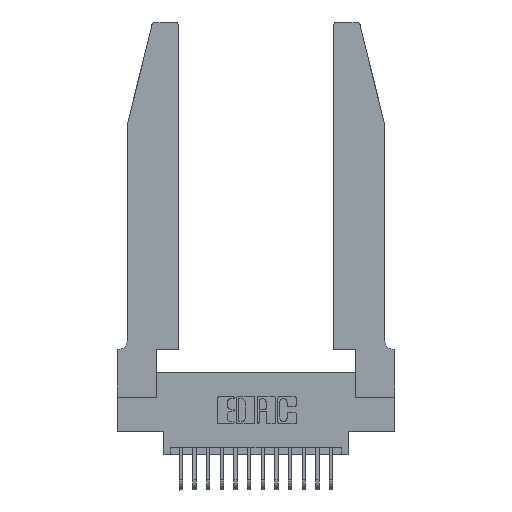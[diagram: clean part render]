
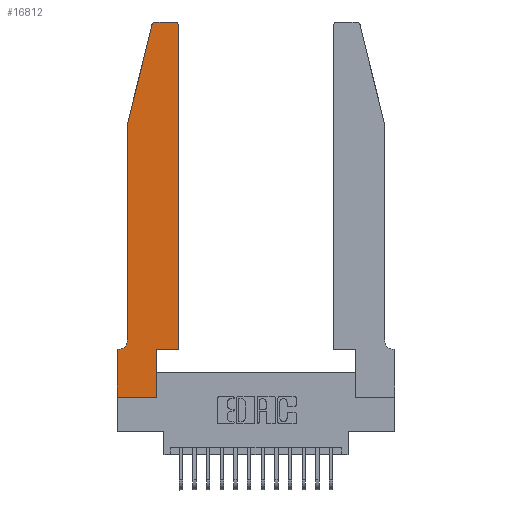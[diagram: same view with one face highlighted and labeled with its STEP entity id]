
A CAD part, top view. The second image highlights one B-rep face of the part: STEP entity #16812.
In plain terms, the highlighted planar face has unit normal (0, 0, 1).
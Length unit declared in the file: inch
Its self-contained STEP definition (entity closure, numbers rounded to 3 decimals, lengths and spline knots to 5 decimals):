
#8 = AXIS2_PLACEMENT_3D ( 'NONE', #12421, #4055, #13852 ) ;
#467 = CARTESIAN_POINT ( 'NONE',  ( 0.25487, 2.72718, 0.37 ) ) ;
#629 = CARTESIAN_POINT ( 'NONE',  ( 0.0755, 2., 0.37 ) ) ;
#680 = ORIENTED_EDGE ( 'NONE', *, *, #9039, .T. ) ;
#1003 = EDGE_CURVE ( 'NONE', #6832, #10895, #7825, .T. ) ;
#1059 = DIRECTION ( 'NONE',  ( 0., 0., 1. ) ) ;
#1195 = VERTEX_POINT ( 'NONE', #1976 ) ;
#1223 = VECTOR ( 'NONE', #12693, 39.37008 ) ;
#1253 = CARTESIAN_POINT ( 'NONE',  ( 0.4505, 0.35, 0.37 ) ) ;
#1284 = ORIENTED_EDGE ( 'NONE', *, *, #8833, .T. ) ;
#1319 = CARTESIAN_POINT ( 'NONE',  ( 0.4205, 2.72, 0.37 ) ) ;
#1499 = DIRECTION ( 'NONE',  ( -0.239, -0.971, 0. ) ) ;
#1777 = ORIENTED_EDGE ( 'NONE', *, *, #14764, .T. ) ;
#1808 = VERTEX_POINT ( 'NONE', #10094 ) ;
#1976 = CARTESIAN_POINT ( 'NONE',  ( 0.4205, 2.75, 0.37 ) ) ;
#2432 = VECTOR ( 'NONE', #6326, 39.37008 ) ;
#2633 = VERTEX_POINT ( 'NONE', #11540 ) ;
#2663 = EDGE_CURVE ( 'NONE', #10895, #10736, #10654, .T. ) ;
#2741 = DIRECTION ( 'NONE',  ( 1., 0., 0. ) ) ;
#2870 = CIRCLE ( 'NONE', #10243, 0.03 ) ;
#3217 = CARTESIAN_POINT ( 'NONE',  ( 0.4505, 0.35, 0.37 ) ) ;
#3336 = ORIENTED_EDGE ( 'NONE', *, *, #1003, .T. ) ;
#3367 = CARTESIAN_POINT ( 'NONE',  ( 0., 0., 0.37 ) ) ;
#3720 = EDGE_CURVE ( 'NONE', #6846, #8641, #5545, .T. ) ;
#3781 = LINE ( 'NONE', #14491, #10805 ) ;
#4012 = VECTOR ( 'NONE', #1499, 39.37008 ) ;
#4055 = DIRECTION ( 'NONE',  ( 0., 0., 1. ) ) ;
#4459 = LINE ( 'NONE', #11318, #4012 ) ;
#4908 = CARTESIAN_POINT ( 'NONE',  ( 0.4505, 0.35, 0.37 ) ) ;
#4925 = LINE ( 'NONE', #17591, #8196 ) ;
#5019 = CARTESIAN_POINT ( 'NONE',  ( 0., 0., 0.37 ) ) ;
#5020 = EDGE_CURVE ( 'NONE', #13563, #1195, #2870, .T. ) ;
#5200 = CIRCLE ( 'NONE', #8, 0.03 ) ;
#5247 = ORIENTED_EDGE ( 'NONE', *, *, #12116, .T. ) ;
#5545 = CIRCLE ( 'NONE', #12498, 0.07 ) ;
#6326 = DIRECTION ( 'NONE',  ( 0., 1., 0. ) ) ;
#6387 = ORIENTED_EDGE ( 'NONE', *, *, #9417, .T. ) ;
#6499 = LINE ( 'NONE', #3367, #16728 ) ;
#6832 = VERTEX_POINT ( 'NONE', #13733 ) ;
#6846 = VERTEX_POINT ( 'NONE', #9599 ) ;
#7825 = LINE ( 'NONE', #14633, #1223 ) ;
#7888 = DIRECTION ( 'NONE',  ( -1., 0., 0. ) ) ;
#8196 = VECTOR ( 'NONE', #7888, 39.37008 ) ;
#8377 = CARTESIAN_POINT ( 'NONE',  ( 0.0055, 0.42, 0.37 ) ) ;
#8641 = VERTEX_POINT ( 'NONE', #11589 ) ;
#8833 = EDGE_CURVE ( 'NONE', #8641, #11203, #13566, .T. ) ;
#8987 = AXIS2_PLACEMENT_3D ( 'NONE', #9490, #1059, #10892 ) ;
#9039 = EDGE_CURVE ( 'NONE', #1808, #11910, #5200, .T. ) ;
#9086 = LINE ( 'NONE', #5019, #15621 ) ;
#9417 = EDGE_CURVE ( 'NONE', #11203, #2633, #6499, .T. ) ;
#9490 = CARTESIAN_POINT ( 'NONE',  ( 0., 0.35, 0.37 ) ) ;
#9497 = EDGE_LOOP ( 'NONE', ( #17051, #680, #12444, #5247, #14011, #1284, #6387, #1777, #3336, #10221, #10438, #15883 ) ) ;
#9599 = CARTESIAN_POINT ( 'NONE',  ( 0.0755, 0.42, 0.37 ) ) ;
#9829 = DIRECTION ( 'NONE',  ( -1., 0., 0. ) ) ;
#9876 = VECTOR ( 'NONE', #12005, 39.37008 ) ;
#10094 = CARTESIAN_POINT ( 'NONE',  ( 0.284, 2.75, 0.37 ) ) ;
#10221 = ORIENTED_EDGE ( 'NONE', *, *, #2663, .T. ) ;
#10243 = AXIS2_PLACEMENT_3D ( 'NONE', #1319, #11147, #2741 ) ;
#10438 = ORIENTED_EDGE ( 'NONE', *, *, #17857, .T. ) ;
#10599 = EDGE_CURVE ( 'NONE', #1195, #1808, #4925, .T. ) ;
#10654 = LINE ( 'NONE', #3217, #17549 ) ;
#10736 = VERTEX_POINT ( 'NONE', #1253 ) ;
#10805 = VECTOR ( 'NONE', #15880, 39.37008 ) ;
#10838 = DIRECTION ( 'NONE',  ( 1., 0., 0. ) ) ;
#10892 = DIRECTION ( 'NONE',  ( 1., 0., 0. ) ) ;
#10895 = VERTEX_POINT ( 'NONE', #15824 ) ;
#10966 = VERTEX_POINT ( 'NONE', #629 ) ;
#11147 = DIRECTION ( 'NONE',  ( 0., 0., 1. ) ) ;
#11203 = VERTEX_POINT ( 'NONE', #15268 ) ;
#11318 = CARTESIAN_POINT ( 'NONE',  ( 0.0755, 2., 0.37 ) ) ;
#11540 = CARTESIAN_POINT ( 'NONE',  ( 0., 0., 0.37 ) ) ;
#11589 = CARTESIAN_POINT ( 'NONE',  ( 0.0055, 0.35, 0.37 ) ) ;
#11716 = CARTESIAN_POINT ( 'NONE',  ( 0.4505, 2.72, 0.37 ) ) ;
#11824 = EDGE_CURVE ( 'NONE', #11910, #10966, #4459, .T. ) ;
#11910 = VERTEX_POINT ( 'NONE', #467 ) ;
#12005 = DIRECTION ( 'NONE',  ( -1., 0., 0. ) ) ;
#12116 = EDGE_CURVE ( 'NONE', #10966, #6846, #3781, .T. ) ;
#12421 = CARTESIAN_POINT ( 'NONE',  ( 0.284, 2.72, 0.37 ) ) ;
#12444 = ORIENTED_EDGE ( 'NONE', *, *, #11824, .T. ) ;
#12498 = AXIS2_PLACEMENT_3D ( 'NONE', #8377, #18062, #9829 ) ;
#12547 = FACE_OUTER_BOUND ( 'NONE', #9497, .T. ) ;
#12693 = DIRECTION ( 'NONE',  ( 0., 1., 0. ) ) ;
#13221 = DIRECTION ( 'NONE',  ( 0., -1., 0. ) ) ;
#13563 = VERTEX_POINT ( 'NONE', #11716 ) ;
#13566 = LINE ( 'NONE', #17497, #9876 ) ;
#13622 = LINE ( 'NONE', #4908, #2432 ) ;
#13733 = CARTESIAN_POINT ( 'NONE',  ( 0.2865, 0., 0.37 ) ) ;
#13852 = DIRECTION ( 'NONE',  ( 1., 0., 0. ) ) ;
#14011 = ORIENTED_EDGE ( 'NONE', *, *, #3720, .T. ) ;
#14443 = DIRECTION ( 'NONE',  ( 1., 0., 0. ) ) ;
#14491 = CARTESIAN_POINT ( 'NONE',  ( 0.0755, 2., 0.37 ) ) ;
#14633 = CARTESIAN_POINT ( 'NONE',  ( 0.2865, 0.35, 0.37 ) ) ;
#14764 = EDGE_CURVE ( 'NONE', #2633, #6832, #9086, .T. ) ;
#15268 = CARTESIAN_POINT ( 'NONE',  ( 0., 0.35, 0.37 ) ) ;
#15621 = VECTOR ( 'NONE', #10838, 39.37008 ) ;
#15824 = CARTESIAN_POINT ( 'NONE',  ( 0.2865, 0.35, 0.37 ) ) ;
#15880 = DIRECTION ( 'NONE',  ( 0., -1., 0. ) ) ;
#15883 = ORIENTED_EDGE ( 'NONE', *, *, #5020, .T. ) ;
#16728 = VECTOR ( 'NONE', #13221, 39.37008 ) ;
#16812 = ADVANCED_FACE ( 'NONE', ( #12547 ), #17754, .T. ) ;
#17051 = ORIENTED_EDGE ( 'NONE', *, *, #10599, .T. ) ;
#17497 = CARTESIAN_POINT ( 'NONE',  ( 0.0755, 0.35, 0.37 ) ) ;
#17549 = VECTOR ( 'NONE', #14443, 39.37008 ) ;
#17591 = CARTESIAN_POINT ( 'NONE',  ( 0.2605, 2.75, 0.37 ) ) ;
#17754 = PLANE ( 'NONE',  #8987 ) ;
#17857 = EDGE_CURVE ( 'NONE', #10736, #13563, #13622, .T. ) ;
#18062 = DIRECTION ( 'NONE',  ( 0., 0., -1. ) ) ;
